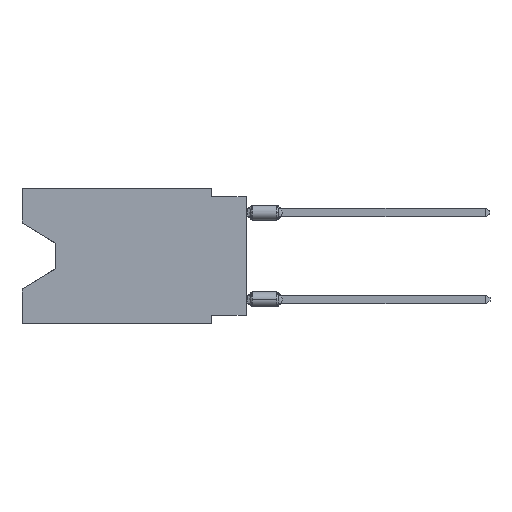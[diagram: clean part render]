
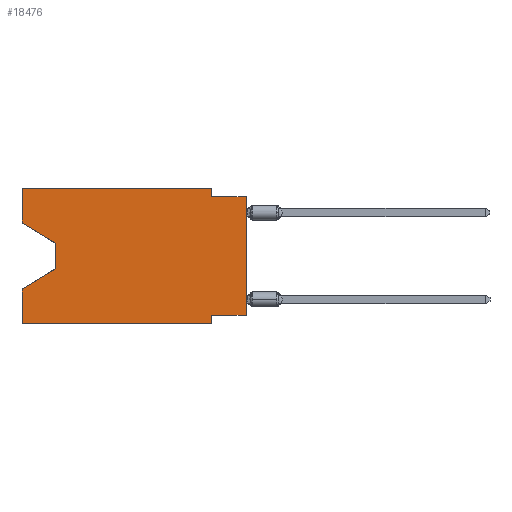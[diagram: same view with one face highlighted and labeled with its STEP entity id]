
A CAD part, left-side view. The second image highlights one B-rep face of the part: STEP entity #18476.
In plain terms, the highlighted planar face has unit normal (-1, 0, 0).
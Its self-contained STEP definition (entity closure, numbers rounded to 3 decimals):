
#57 = EDGE_CURVE ( 'NONE', #14321, #3023, #17972, .T. ) ;
#382 = ORIENTED_EDGE ( 'NONE', *, *, #19686, .T. ) ;
#1355 = EDGE_LOOP ( 'NONE', ( #382, #15244, #10697, #5677, #13416, #21139, #19431, #12752, #15592, #6181, #3453, #7701 ) ) ;
#1588 = DIRECTION ( 'NONE',  ( 0., 0., 1. ) ) ;
#1610 = VERTEX_POINT ( 'NONE', #9871 ) ;
#1937 = EDGE_CURVE ( 'NONE', #21892, #14321, #11393, .T. ) ;
#1969 = LINE ( 'NONE', #5857, #20669 ) ;
#2169 = CARTESIAN_POINT ( 'NONE',  ( 0., 2.54, 0. ) ) ;
#2512 = VECTOR ( 'NONE', #6080, 1000. ) ;
#3023 = VERTEX_POINT ( 'NONE', #19354 ) ;
#3263 = DIRECTION ( 'NONE',  ( 0., 0., -1. ) ) ;
#3294 = VECTOR ( 'NONE', #6155, 1000. ) ;
#3453 = ORIENTED_EDGE ( 'NONE', *, *, #3748, .F. ) ;
#3738 = CARTESIAN_POINT ( 'NONE',  ( 0., 0., -0.635 ) ) ;
#3748 = EDGE_CURVE ( 'NONE', #18278, #7945, #8282, .T. ) ;
#3953 = CARTESIAN_POINT ( 'NONE',  ( 0., 0., 0. ) ) ;
#3982 = EDGE_CURVE ( 'NONE', #5206, #9502, #9428, .T. ) ;
#4102 = EDGE_CURVE ( 'NONE', #11736, #25563, #15653, .T. ) ;
#4869 = CARTESIAN_POINT ( 'NONE',  ( 0., 13.97, -5.893 ) ) ;
#5206 = VERTEX_POINT ( 'NONE', #10064 ) ;
#5378 = DIRECTION ( 'NONE',  ( 1., 0., 0. ) ) ;
#5677 = ORIENTED_EDGE ( 'NONE', *, *, #15395, .F. ) ;
#5715 = VECTOR ( 'NONE', #19446, 1000. ) ;
#5857 = CARTESIAN_POINT ( 'NONE',  ( 0., 16.383, 0. ) ) ;
#6060 = EDGE_CURVE ( 'NONE', #9470, #18278, #16063, .T. ) ;
#6080 = DIRECTION ( 'NONE',  ( 0., 0., 1. ) ) ;
#6155 = DIRECTION ( 'NONE',  ( 0., 0., -1. ) ) ;
#6181 = ORIENTED_EDGE ( 'NONE', *, *, #11732, .F. ) ;
#6345 = CARTESIAN_POINT ( 'NONE',  ( 0., 16.383, 0. ) ) ;
#6873 = CARTESIAN_POINT ( 'NONE',  ( 0., 13.97, -4.013 ) ) ;
#7204 = LINE ( 'NONE', #25480, #9006 ) ;
#7432 = DIRECTION ( 'NONE',  ( 0., 0., -1. ) ) ;
#7701 = ORIENTED_EDGE ( 'NONE', *, *, #6060, .F. ) ;
#7764 = CARTESIAN_POINT ( 'NONE',  ( 0., 16.383, 0. ) ) ;
#7773 = VECTOR ( 'NONE', #21109, 1000. ) ;
#7945 = VERTEX_POINT ( 'NONE', #2169 ) ;
#8115 = DIRECTION ( 'NONE',  ( 0., -1., 0. ) ) ;
#8183 = VECTOR ( 'NONE', #3263, 1000. ) ;
#8276 = CARTESIAN_POINT ( 'NONE',  ( 0., 0., -9.271 ) ) ;
#8282 = LINE ( 'NONE', #6345, #16487 ) ;
#9006 = VECTOR ( 'NONE', #8115, 1000. ) ;
#9281 = CARTESIAN_POINT ( 'NONE',  ( 0., 2.54, -9.271 ) ) ;
#9428 = LINE ( 'NONE', #3738, #7773 ) ;
#9470 = VERTEX_POINT ( 'NONE', #17057 ) ;
#9502 = VERTEX_POINT ( 'NONE', #15367 ) ;
#9871 = CARTESIAN_POINT ( 'NONE',  ( 0., 13.97, -4.013 ) ) ;
#10064 = CARTESIAN_POINT ( 'NONE',  ( 0., 2.54, -0.635 ) ) ;
#10294 = CARTESIAN_POINT ( 'NONE',  ( 0., 16.383, -7.36 ) ) ;
#10348 = VECTOR ( 'NONE', #11722, 1000. ) ;
#10697 = ORIENTED_EDGE ( 'NONE', *, *, #4102, .T. ) ;
#11256 = CARTESIAN_POINT ( 'NONE',  ( 0., 16.383, -9.906 ) ) ;
#11393 = LINE ( 'NONE', #15543, #5715 ) ;
#11452 = DIRECTION ( 'NONE',  ( 0., -0.855, -0.519 ) ) ;
#11722 = DIRECTION ( 'NONE',  ( 0., 0., 1. ) ) ;
#11732 = EDGE_CURVE ( 'NONE', #7945, #5206, #12388, .T. ) ;
#11736 = VERTEX_POINT ( 'NONE', #4869 ) ;
#12388 = LINE ( 'NONE', #20559, #21808 ) ;
#12752 = ORIENTED_EDGE ( 'NONE', *, *, #16265, .T. ) ;
#13416 = ORIENTED_EDGE ( 'NONE', *, *, #21000, .T. ) ;
#13848 = DIRECTION ( 'NONE',  ( 0., 0.855, -0.519 ) ) ;
#13853 = EDGE_CURVE ( 'NONE', #1610, #11736, #24748, .T. ) ;
#14321 = VERTEX_POINT ( 'NONE', #9281 ) ;
#15244 = ORIENTED_EDGE ( 'NONE', *, *, #13853, .T. ) ;
#15367 = CARTESIAN_POINT ( 'NONE',  ( 0., 0., -0.635 ) ) ;
#15395 = EDGE_CURVE ( 'NONE', #20509, #25563, #1969, .T. ) ;
#15543 = CARTESIAN_POINT ( 'NONE',  ( 0., 0., -9.271 ) ) ;
#15592 = ORIENTED_EDGE ( 'NONE', *, *, #3982, .F. ) ;
#15653 = LINE ( 'NONE', #23556, #18151 ) ;
#15741 = LINE ( 'NONE', #3953, #10348 ) ;
#16063 = LINE ( 'NONE', #19960, #2512 ) ;
#16265 = EDGE_CURVE ( 'NONE', #21892, #9502, #15741, .T. ) ;
#16487 = VECTOR ( 'NONE', #20217, 1000. ) ;
#16703 = AXIS2_PLACEMENT_3D ( 'NONE', #25442, #5378, #7432 ) ;
#17057 = CARTESIAN_POINT ( 'NONE',  ( 0., 16.383, -2.546 ) ) ;
#17316 = CARTESIAN_POINT ( 'NONE',  ( 0., 16.383, -2.546 ) ) ;
#17972 = LINE ( 'NONE', #22103, #3294 ) ;
#18151 = VECTOR ( 'NONE', #13848, 1000. ) ;
#18278 = VERTEX_POINT ( 'NONE', #7764 ) ;
#18476 = ADVANCED_FACE ( 'NONE', ( #19371 ), #23251, .F. ) ;
#19354 = CARTESIAN_POINT ( 'NONE',  ( 0., 2.54, -9.906 ) ) ;
#19371 = FACE_OUTER_BOUND ( 'NONE', #1355, .T. ) ;
#19431 = ORIENTED_EDGE ( 'NONE', *, *, #1937, .F. ) ;
#19446 = DIRECTION ( 'NONE',  ( 0., 1., 0. ) ) ;
#19686 = EDGE_CURVE ( 'NONE', #9470, #1610, #21451, .T. ) ;
#19960 = CARTESIAN_POINT ( 'NONE',  ( 0., 16.383, 0. ) ) ;
#20217 = DIRECTION ( 'NONE',  ( 0., -1., 0. ) ) ;
#20273 = VECTOR ( 'NONE', #11452, 1000. ) ;
#20318 = DIRECTION ( 'NONE',  ( 0., 0., -1. ) ) ;
#20509 = VERTEX_POINT ( 'NONE', #11256 ) ;
#20559 = CARTESIAN_POINT ( 'NONE',  ( 0., 2.54, 0. ) ) ;
#20669 = VECTOR ( 'NONE', #1588, 1000. ) ;
#21000 = EDGE_CURVE ( 'NONE', #20509, #3023, #7204, .T. ) ;
#21109 = DIRECTION ( 'NONE',  ( 0., -1., 0. ) ) ;
#21139 = ORIENTED_EDGE ( 'NONE', *, *, #57, .F. ) ;
#21451 = LINE ( 'NONE', #17316, #20273 ) ;
#21808 = VECTOR ( 'NONE', #20318, 1000. ) ;
#21892 = VERTEX_POINT ( 'NONE', #8276 ) ;
#22103 = CARTESIAN_POINT ( 'NONE',  ( 0., 2.54, -9.906 ) ) ;
#23251 = PLANE ( 'NONE',  #16703 ) ;
#23556 = CARTESIAN_POINT ( 'NONE',  ( 0., 13.97, -5.893 ) ) ;
#24748 = LINE ( 'NONE', #6873, #8183 ) ;
#25442 = CARTESIAN_POINT ( 'NONE',  ( 0., 16.383, 0. ) ) ;
#25480 = CARTESIAN_POINT ( 'NONE',  ( 0., 16.383, -9.906 ) ) ;
#25563 = VERTEX_POINT ( 'NONE', #10294 ) ;
